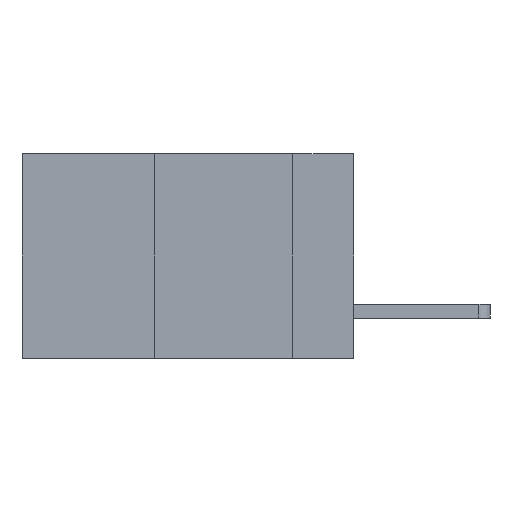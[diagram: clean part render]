
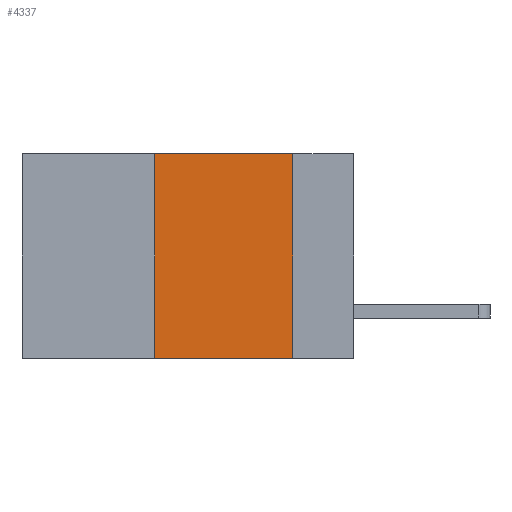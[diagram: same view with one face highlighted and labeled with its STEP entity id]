
A CAD part, left-side view. The second image highlights one B-rep face of the part: STEP entity #4337.
In plain terms, the highlighted planar face has unit normal (-1, 0, 0).
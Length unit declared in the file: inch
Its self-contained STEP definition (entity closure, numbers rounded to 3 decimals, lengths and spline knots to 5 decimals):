
#182 = CARTESIAN_POINT ( 'NONE',  ( 0., 0.11, 0. ) ) ;
#235 = EDGE_CURVE ( 'NONE', #9722, #6275, #2060, .T. ) ;
#489 = EDGE_LOOP ( 'NONE', ( #4295, #1691, #1769, #10402 ) ) ;
#530 = CARTESIAN_POINT ( 'NONE',  ( 0., 0.36, 0. ) ) ;
#757 = DIRECTION ( 'NONE',  ( 0., 0., -1. ) ) ;
#1351 = VECTOR ( 'NONE', #10011, 39.37008 ) ;
#1615 = DIRECTION ( 'NONE',  ( 0., 0., 1. ) ) ;
#1691 = ORIENTED_EDGE ( 'NONE', *, *, #2166, .F. ) ;
#1769 = ORIENTED_EDGE ( 'NONE', *, *, #235, .F. ) ;
#2060 = LINE ( 'NONE', #9134, #6880 ) ;
#2166 = EDGE_CURVE ( 'NONE', #6275, #3049, #8134, .T. ) ;
#2939 = FACE_OUTER_BOUND ( 'NONE', #489, .T. ) ;
#3049 = VERTEX_POINT ( 'NONE', #182 ) ;
#3166 = EDGE_CURVE ( 'NONE', #9722, #6316, #9411, .T. ) ;
#3670 = VECTOR ( 'NONE', #8606, 39.37008 ) ;
#4238 = CARTESIAN_POINT ( 'NONE',  ( 0., 0.6, -0.37 ) ) ;
#4245 = AXIS2_PLACEMENT_3D ( 'NONE', #6401, #6901, #757 ) ;
#4295 = ORIENTED_EDGE ( 'NONE', *, *, #10204, .F. ) ;
#4337 = ADVANCED_FACE ( 'NONE', ( #2939 ), #6432, .F. ) ;
#4475 = CARTESIAN_POINT ( 'NONE',  ( 0., 0.11, 0. ) ) ;
#5107 = CARTESIAN_POINT ( 'NONE',  ( 0., 0.6, 0. ) ) ;
#6135 = DIRECTION ( 'NONE',  ( 0., -1., 0. ) ) ;
#6275 = VERTEX_POINT ( 'NONE', #530 ) ;
#6316 = VERTEX_POINT ( 'NONE', #9244 ) ;
#6401 = CARTESIAN_POINT ( 'NONE',  ( 0., 0.6, 0. ) ) ;
#6432 = PLANE ( 'NONE',  #4245 ) ;
#6880 = VECTOR ( 'NONE', #1615, 39.37008 ) ;
#6901 = DIRECTION ( 'NONE',  ( 1., 0., 0. ) ) ;
#7872 = LINE ( 'NONE', #4475, #1351 ) ;
#8134 = LINE ( 'NONE', #5107, #3670 ) ;
#8606 = DIRECTION ( 'NONE',  ( 0., -1., 0. ) ) ;
#9134 = CARTESIAN_POINT ( 'NONE',  ( 0., 0.36, 0. ) ) ;
#9171 = VECTOR ( 'NONE', #6135, 39.37008 ) ;
#9244 = CARTESIAN_POINT ( 'NONE',  ( 0., 0.11, -0.37 ) ) ;
#9411 = LINE ( 'NONE', #4238, #9171 ) ;
#9722 = VERTEX_POINT ( 'NONE', #10081 ) ;
#10011 = DIRECTION ( 'NONE',  ( 0., 0., -1. ) ) ;
#10081 = CARTESIAN_POINT ( 'NONE',  ( 0., 0.36, -0.37 ) ) ;
#10204 = EDGE_CURVE ( 'NONE', #3049, #6316, #7872, .T. ) ;
#10402 = ORIENTED_EDGE ( 'NONE', *, *, #3166, .T. ) ;
